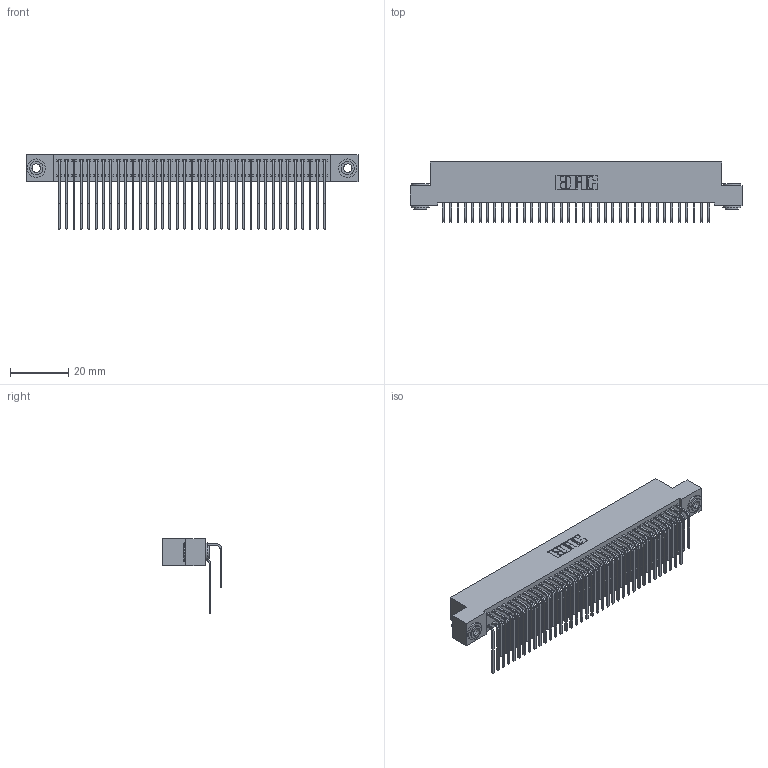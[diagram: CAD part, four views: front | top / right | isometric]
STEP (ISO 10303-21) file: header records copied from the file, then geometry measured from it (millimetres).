
FILE_DESCRIPTION (( 'STEP AP203' ), '1' );
FILE_NAME ('342-074-559-203.STEP', '2018-08-13T11:52:26', ( '' ), ( '' ), 'SwSTEP 2.0', 'SolidWorks 2016', '' );
FILE_SCHEMA (( 'CONFIG_CONTROL_DESIGN' ));
Length unit declared in the file: inch
Products named in the file (5): 342-074-559-203; 342 Part_.156 TH; 345-292-001_558 559 Tail - 1; 345-292-001_559 Tail - 2; 342-250-002_345-250-002-102
Assembly tree (77 placements, depth 2):
  342-074-559-203
    342 Part_.156 TH
    345-292-001_558 559 Tail - 1  x37
    345-292-001_559 Tail - 2  x37
    342-250-002_345-250-002-102  x2
Bounding box: 114.3 x 20.64 x 25.78 mm (x, y, z)
Volume: 10695.9 mm3; surface area: 19432.2 mm2
Topology: 77 solids, 77 shells, 4144 faces, 12289 edges, 8090 vertices
Faces by surface type: plane 2888, cylinder 1248, cone 8
Entity records: 26752 total; most frequent: CARTESIAN_POINT 4464, ORIENTED_EDGE 4342, DIRECTION 3837, EDGE_CURVE 2171, LINE 1979, VECTOR 1979, VERTEX_POINT 1442, AXIS2_PLACEMENT_3D 929
